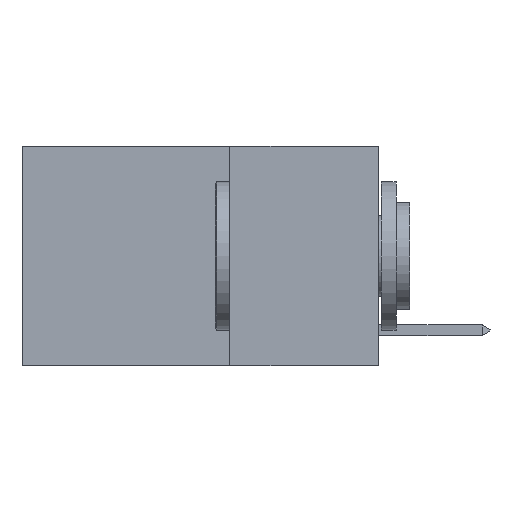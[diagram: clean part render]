
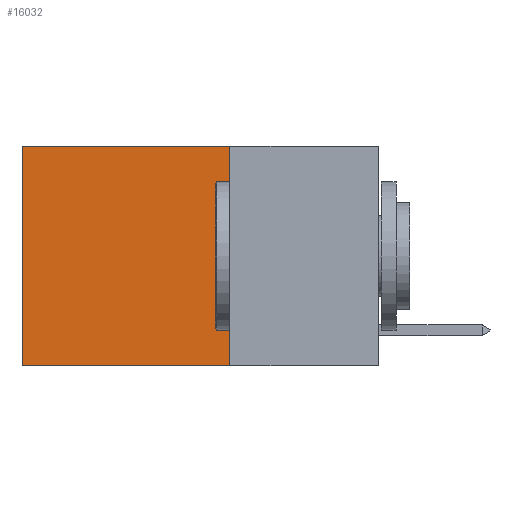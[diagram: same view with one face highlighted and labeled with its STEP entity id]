
A CAD part, left-side view. The second image highlights one B-rep face of the part: STEP entity #16032.
In plain terms, the highlighted planar face has unit normal (-1, 0, 0).
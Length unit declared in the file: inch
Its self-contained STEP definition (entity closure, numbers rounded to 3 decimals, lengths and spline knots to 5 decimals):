
#126 = EDGE_CURVE ( 'NONE', #12292, #10755, #16270, .T. ) ;
#1147 = EDGE_CURVE ( 'NONE', #19692, #3318, #11909, .T. ) ;
#1616 = CARTESIAN_POINT ( 'NONE',  ( 0.2625, 0.25, 0. ) ) ;
#2591 = CARTESIAN_POINT ( 'NONE',  ( 0.2625, 0.25, 0. ) ) ;
#2820 = VECTOR ( 'NONE', #15851, 39.37008 ) ;
#3139 = ORIENTED_EDGE ( 'NONE', *, *, #8205, .F. ) ;
#3161 = AXIS2_PLACEMENT_3D ( 'NONE', #1616, #5061, #16190 ) ;
#3318 = VERTEX_POINT ( 'NONE', #15432 ) ;
#3320 = DIRECTION ( 'NONE',  ( 0., 0., -1. ) ) ;
#3489 = CARTESIAN_POINT ( 'NONE',  ( 0.2625, 0.25, 0. ) ) ;
#3859 = LINE ( 'NONE', #4675, #2820 ) ;
#4505 = CARTESIAN_POINT ( 'NONE',  ( 0.2625, 0.25, 0. ) ) ;
#4675 = CARTESIAN_POINT ( 'NONE',  ( 0.2625, 0.25, -0.37 ) ) ;
#5061 = DIRECTION ( 'NONE',  ( 1., 0., 0. ) ) ;
#5397 = ORIENTED_EDGE ( 'NONE', *, *, #1147, .F. ) ;
#6207 = DIRECTION ( 'NONE',  ( 0., 1., 0. ) ) ;
#6537 = VECTOR ( 'NONE', #6207, 39.37008 ) ;
#6554 = EDGE_CURVE ( 'NONE', #19692, #12292, #18963, .T. ) ;
#6596 = VECTOR ( 'NONE', #3320, 39.37008 ) ;
#7667 = DIRECTION ( 'NONE',  ( 0., 0., -1. ) ) ;
#8205 = EDGE_CURVE ( 'NONE', #3318, #10755, #3859, .T. ) ;
#8619 = CARTESIAN_POINT ( 'NONE',  ( 0.2625, 0.6, 0. ) ) ;
#9883 = CARTESIAN_POINT ( 'NONE',  ( 0.2625, 0.6, -0.37 ) ) ;
#10755 = VERTEX_POINT ( 'NONE', #9883 ) ;
#11909 = LINE ( 'NONE', #3489, #6596 ) ;
#12198 = VECTOR ( 'NONE', #7667, 39.37008 ) ;
#12292 = VERTEX_POINT ( 'NONE', #13824 ) ;
#13122 = ORIENTED_EDGE ( 'NONE', *, *, #126, .T. ) ;
#13824 = CARTESIAN_POINT ( 'NONE',  ( 0.2625, 0.6, 0. ) ) ;
#14691 = PLANE ( 'NONE',  #3161 ) ;
#15122 = EDGE_LOOP ( 'NONE', ( #13122, #3139, #5397, #15800 ) ) ;
#15432 = CARTESIAN_POINT ( 'NONE',  ( 0.2625, 0.25, -0.37 ) ) ;
#15800 = ORIENTED_EDGE ( 'NONE', *, *, #6554, .T. ) ;
#15851 = DIRECTION ( 'NONE',  ( 0., 1., 0. ) ) ;
#16032 = ADVANCED_FACE ( 'NONE', ( #18399 ), #14691, .F. ) ;
#16190 = DIRECTION ( 'NONE',  ( 0., 0., -1. ) ) ;
#16270 = LINE ( 'NONE', #8619, #12198 ) ;
#18399 = FACE_OUTER_BOUND ( 'NONE', #15122, .T. ) ;
#18963 = LINE ( 'NONE', #4505, #6537 ) ;
#19692 = VERTEX_POINT ( 'NONE', #2591 ) ;
